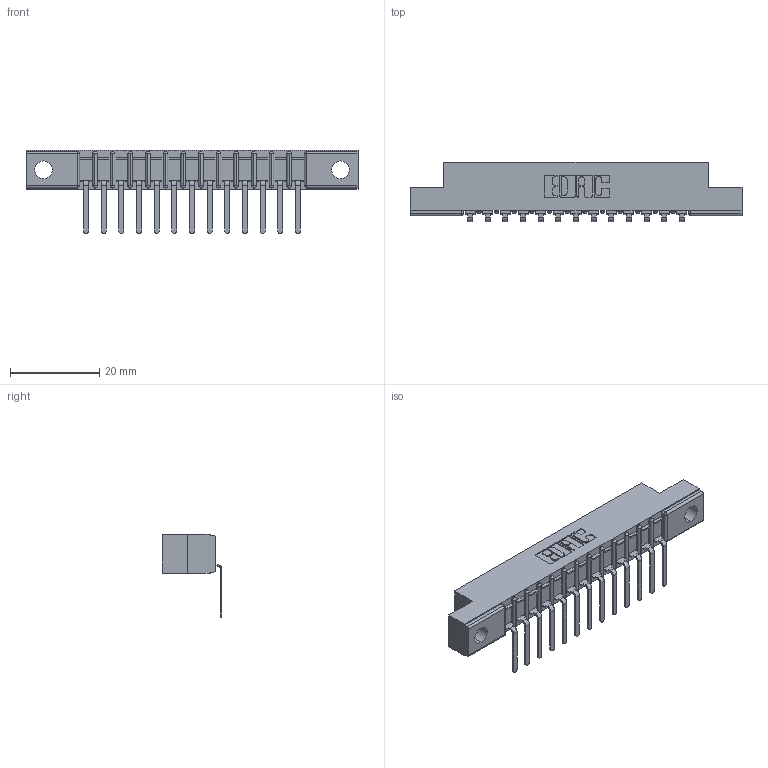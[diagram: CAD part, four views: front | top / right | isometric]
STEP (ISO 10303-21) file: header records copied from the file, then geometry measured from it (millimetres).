
FILE_DESCRIPTION (( 'STEP AP203' ), '1' );
FILE_NAME ('357-013-457-102.STEP', '2020-09-30T14:46:58', ( '' ), ( '' ), 'SwSTEP 2.0', 'SolidWorks 2020', '' );
FILE_SCHEMA (( 'CONFIG_CONTROL_DESIGN' ));
Length unit declared in the file: inch
Products named in the file (3): 357-013-457-102; 307-290-002_557; 307 Part_.128 Dia Mounting Holes
Assembly tree (14 placements, depth 2):
  357-013-457-102
    307 Part_.128 Dia Mounting Holes
    307-290-002_557  x13
Bounding box: 74.52 x 13.32 x 18.67 mm (x, y, z)
Volume: 4862.4 mm3; surface area: 8406 mm2
Topology: 14 solids, 14 shells, 1146 faces, 3495 edges, 2290 vertices
Faces by surface type: plane 681, cylinder 437, sphere 28
Entity records: 15576 total; most frequent: CARTESIAN_POINT 2624, ORIENTED_EDGE 2614, DIRECTION 2563, EDGE_CURVE 1307, VECTOR 985, LINE 985, VERTEX_POINT 850, AXIS2_PLACEMENT_3D 789
